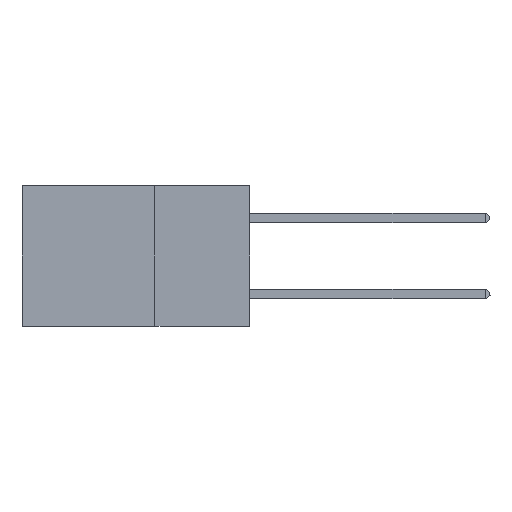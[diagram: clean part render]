
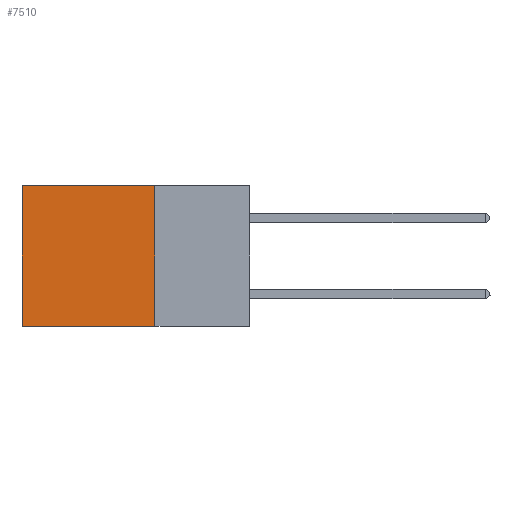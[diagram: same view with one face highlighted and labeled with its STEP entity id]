
A CAD part, left-side view. The second image highlights one B-rep face of the part: STEP entity #7510.
In plain terms, the highlighted planar face has unit normal (-1, 0, 0).
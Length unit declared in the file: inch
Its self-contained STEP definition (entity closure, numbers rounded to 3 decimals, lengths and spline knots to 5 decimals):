
#451 = VERTEX_POINT ( 'NONE', #9951 ) ;
#839 = VECTOR ( 'NONE', #1579, 39.37008 ) ;
#936 = LINE ( 'NONE', #12333, #11026 ) ;
#1295 = VECTOR ( 'NONE', #12239, 39.37008 ) ;
#1579 = DIRECTION ( 'NONE',  ( 0., 0., -1. ) ) ;
#1892 = EDGE_LOOP ( 'NONE', ( #15377, #5862, #11563, #15594 ) ) ;
#4108 = DIRECTION ( 'NONE',  ( 1., 0., 0. ) ) ;
#4419 = LINE ( 'NONE', #10177, #839 ) ;
#5053 = CARTESIAN_POINT ( 'NONE',  ( 0.2875, 0.25, 0. ) ) ;
#5862 = ORIENTED_EDGE ( 'NONE', *, *, #7620, .F. ) ;
#6470 = CARTESIAN_POINT ( 'NONE',  ( 0.2875, 0.6, 0. ) ) ;
#7510 = ADVANCED_FACE ( 'NONE', ( #8791 ), #12277, .F. ) ;
#7620 = EDGE_CURVE ( 'NONE', #451, #16816, #936, .T. ) ;
#7897 = VERTEX_POINT ( 'NONE', #6470 ) ;
#7902 = DIRECTION ( 'NONE',  ( 0., 1., 0. ) ) ;
#8079 = CARTESIAN_POINT ( 'NONE',  ( 0.2875, 0.25, 0. ) ) ;
#8089 = VECTOR ( 'NONE', #10574, 39.37008 ) ;
#8791 = FACE_OUTER_BOUND ( 'NONE', #1892, .T. ) ;
#9687 = CARTESIAN_POINT ( 'NONE',  ( 0.2875, 0.6, -0.37 ) ) ;
#9797 = EDGE_CURVE ( 'NONE', #11088, #7897, #10488, .T. ) ;
#9951 = CARTESIAN_POINT ( 'NONE',  ( 0.2875, 0.25, -0.37 ) ) ;
#10177 = CARTESIAN_POINT ( 'NONE',  ( 0.2875, 0.25, 0. ) ) ;
#10488 = LINE ( 'NONE', #12165, #1295 ) ;
#10574 = DIRECTION ( 'NONE',  ( 0., 0., -1. ) ) ;
#10956 = EDGE_CURVE ( 'NONE', #11088, #451, #4419, .T. ) ;
#11026 = VECTOR ( 'NONE', #7902, 39.37008 ) ;
#11088 = VERTEX_POINT ( 'NONE', #5053 ) ;
#11563 = ORIENTED_EDGE ( 'NONE', *, *, #10956, .F. ) ;
#12165 = CARTESIAN_POINT ( 'NONE',  ( 0.2875, 0.25, 0. ) ) ;
#12239 = DIRECTION ( 'NONE',  ( 0., 1., 0. ) ) ;
#12277 = PLANE ( 'NONE',  #15450 ) ;
#12333 = CARTESIAN_POINT ( 'NONE',  ( 0.2875, 0.25, -0.37 ) ) ;
#13265 = CARTESIAN_POINT ( 'NONE',  ( 0.2875, 0.6, 0. ) ) ;
#15377 = ORIENTED_EDGE ( 'NONE', *, *, #15990, .T. ) ;
#15450 = AXIS2_PLACEMENT_3D ( 'NONE', #8079, #4108, #15508 ) ;
#15508 = DIRECTION ( 'NONE',  ( 0., 0., -1. ) ) ;
#15594 = ORIENTED_EDGE ( 'NONE', *, *, #9797, .T. ) ;
#15990 = EDGE_CURVE ( 'NONE', #7897, #16816, #16789, .T. ) ;
#16789 = LINE ( 'NONE', #13265, #8089 ) ;
#16816 = VERTEX_POINT ( 'NONE', #9687 ) ;
